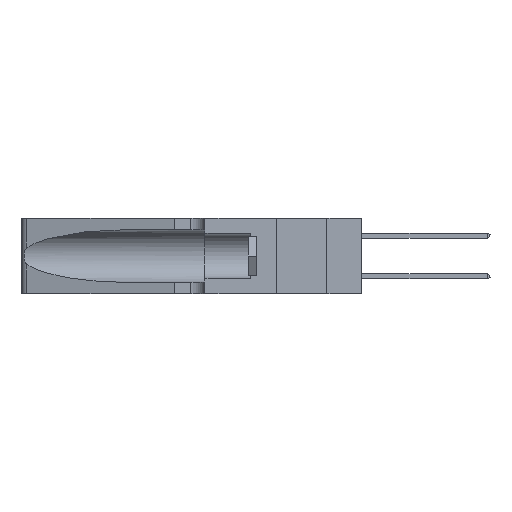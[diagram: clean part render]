
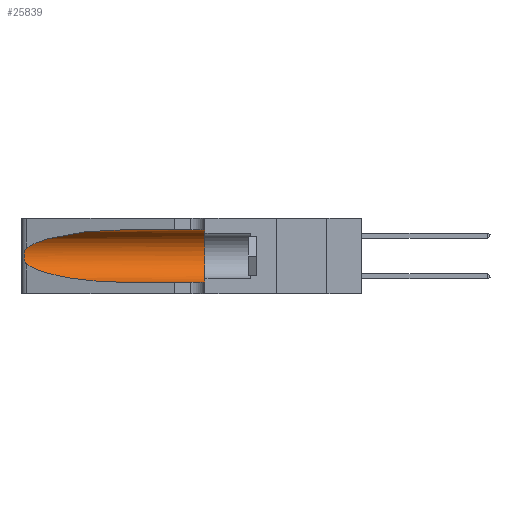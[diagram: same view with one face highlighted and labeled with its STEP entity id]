
A CAD part, left-side view. The second image highlights one B-rep face of the part: STEP entity #25839.
In plain terms, the highlighted cylindrical face has radius 3.308 mm (diameter 6.617 mm), a partial arc.
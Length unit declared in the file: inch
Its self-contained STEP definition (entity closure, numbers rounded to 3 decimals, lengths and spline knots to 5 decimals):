
#1221 = CARTESIAN_POINT ( 'NONE',  ( 0.2373, 1.15595, 0.28018 ) ) ;
#1603 = DIRECTION ( 'NONE',  ( 0., 0., -1. ) ) ;
#2763 = CARTESIAN_POINT ( 'NONE',  ( 0.25854, 1.2359, 0.20912 ) ) ;
#2791 = DIRECTION ( 'NONE',  ( 0., -1., 0. ) ) ;
#3353 = EDGE_LOOP ( 'NONE', ( #34575, #12741, #36280, #5280, #34317, #18163 ) ) ;
#5280 = ORIENTED_EDGE ( 'NONE', *, *, #8085, .T. ) ;
#5352 = VECTOR ( 'NONE', #2791, 39.37008 ) ;
#5541 = VERTEX_POINT ( 'NONE', #17304 ) ;
#5722 = CARTESIAN_POINT ( 'NONE',  ( 0.26075, 1.23896, 0.19203 ) ) ;
#5919 = VERTEX_POINT ( 'NONE', #10292 ) ;
#7194 = FACE_OUTER_BOUND ( 'NONE', #3353, .T. ) ;
#7233 = CARTESIAN_POINT ( 'NONE',  ( 0.1305, 0.35, 0.185 ) ) ;
#7387 = CARTESIAN_POINT ( 'NONE',  ( 0.1305, 1.61858, 0.185 ) ) ;
#7437 = CARTESIAN_POINT ( 'NONE',  ( 0.2373, 1.15595, 0.08982 ) ) ;
#8085 = EDGE_CURVE ( 'NONE', #14605, #11757, #35796, .T. ) ;
#8631 = CARTESIAN_POINT ( 'NONE',  ( 0.26017, 1.23833, 0.17102 ) ) ;
#9462 = VERTEX_POINT ( 'NONE', #19540 ) ;
#10022 = AXIS2_PLACEMENT_3D ( 'NONE', #7233, #27275, #10128 ) ;
#10128 = DIRECTION ( 'NONE',  ( 0., 0., 1. ) ) ;
#10292 = CARTESIAN_POINT ( 'NONE',  ( 0.1305, 0.72297, 0.31525 ) ) ;
#11532 = CARTESIAN_POINT ( 'NONE',  ( 0.25789, 1.23486, 0.15765 ) ) ;
#11757 = VERTEX_POINT ( 'NONE', #12048 ) ;
#12048 = CARTESIAN_POINT ( 'NONE',  ( 0.1305, 0.35, 0.05475 ) ) ;
#12410 =( BOUNDED_CURVE ( )  B_SPLINE_CURVE ( 3, ( #18525, #18650, #1221, #21511 ),
 .UNSPECIFIED., .F., .F. ) 
 B_SPLINE_CURVE_WITH_KNOTS ( ( 4, 4 ),
 ( 1.5708, 2.84003 ),
 .UNSPECIFIED. ) 
 CURVE ( )  GEOMETRIC_REPRESENTATION_ITEM ( )  RATIONAL_B_SPLINE_CURVE ( ( 1., 0.87, 0.87, 1. ) ) 
 REPRESENTATION_ITEM ( '' )  );
#12741 = ORIENTED_EDGE ( 'NONE', *, *, #26076, .T. ) ;
#13222 = CARTESIAN_POINT ( 'NONE',  ( 0.18966, 0.96281, 0.05475 ) ) ;
#13614 = VECTOR ( 'NONE', #18377, 39.37008 ) ;
#14466 = CARTESIAN_POINT ( 'NONE',  ( 0.25555, 1.22993, 0.14849 ) ) ;
#14517 = CARTESIAN_POINT ( 'NONE',  ( 0.1305, 0.72297, 0.05475 ) ) ;
#14605 = VERTEX_POINT ( 'NONE', #14517 ) ;
#17304 = CARTESIAN_POINT ( 'NONE',  ( 0.25487, 1.22718, 0.22369 ) ) ;
#18020 =( BOUNDED_CURVE ( )  B_SPLINE_CURVE ( 3, ( #27490, #7437, #13222, #33171 ),
 .UNSPECIFIED., .F., .F. ) 
 B_SPLINE_CURVE_WITH_KNOTS ( ( 4, 4 ),
 ( 3.44316, 4.71239 ),
 .UNSPECIFIED. ) 
 CURVE ( )  GEOMETRIC_REPRESENTATION_ITEM ( )  RATIONAL_B_SPLINE_CURVE ( ( 1., 0.87, 0.87, 1. ) ) 
 REPRESENTATION_ITEM ( '' )  );
#18163 = ORIENTED_EDGE ( 'NONE', *, *, #24277, .F. ) ;
#18377 = DIRECTION ( 'NONE',  ( 0., -1., 0. ) ) ;
#18525 = CARTESIAN_POINT ( 'NONE',  ( 0.1305, 0.72297, 0.31525 ) ) ;
#18650 = CARTESIAN_POINT ( 'NONE',  ( 0.18966, 0.96281, 0.31525 ) ) ;
#19540 = CARTESIAN_POINT ( 'NONE',  ( 0.1305, 0.35, 0.31525 ) ) ;
#20109 = CARTESIAN_POINT ( 'NONE',  ( 0.25787, 1.23484, 0.2124 ) ) ;
#21511 = CARTESIAN_POINT ( 'NONE',  ( 0.25487, 1.22718, 0.22369 ) ) ;
#21526 = CARTESIAN_POINT ( 'NONE',  ( 0.25487, 1.22718, 0.14631 ) ) ;
#21610 = CYLINDRICAL_SURFACE ( 'NONE', #28870, 0.13025 ) ;
#22972 = CARTESIAN_POINT ( 'NONE',  ( 0.26018, 1.23835, 0.19895 ) ) ;
#23154 = EDGE_CURVE ( 'NONE', #23663, #14605, #18020, .T. ) ;
#23663 = VERTEX_POINT ( 'NONE', #21526 ) ;
#24277 = EDGE_CURVE ( 'NONE', #5919, #9462, #35481, .T. ) ;
#25813 = CARTESIAN_POINT ( 'NONE',  ( 0.26075, 1.23896, 0.178 ) ) ;
#25839 = ADVANCED_FACE ( 'NONE', ( #7194 ), #21610, .F. ) ;
#26076 = EDGE_CURVE ( 'NONE', #5541, #23663, #35783, .T. ) ;
#27275 = DIRECTION ( 'NONE',  ( 0., 1., 0. ) ) ;
#27490 = CARTESIAN_POINT ( 'NONE',  ( 0.25487, 1.22718, 0.14631 ) ) ;
#28556 = CARTESIAN_POINT ( 'NONE',  ( 0.25555, 1.22994, 0.2215 ) ) ;
#28689 = CARTESIAN_POINT ( 'NONE',  ( 0.25856, 1.23593, 0.16098 ) ) ;
#28870 = AXIS2_PLACEMENT_3D ( 'NONE', #7387, #33123, #1603 ) ;
#28955 = EDGE_CURVE ( 'NONE', #5919, #5541, #12410, .T. ) ;
#30147 = CIRCLE ( 'NONE', #10022, 0.13025 ) ;
#31515 = CARTESIAN_POINT ( 'NONE',  ( 0.25639, 1.23186, 0.15144 ) ) ;
#32514 = CARTESIAN_POINT ( 'NONE',  ( 0.1305, 1.61858, 0.31525 ) ) ;
#33123 = DIRECTION ( 'NONE',  ( 0., -1., 0. ) ) ;
#33171 = CARTESIAN_POINT ( 'NONE',  ( 0.1305, 0.72297, 0.05475 ) ) ;
#34137 = CARTESIAN_POINT ( 'NONE',  ( 0.25487, 1.22718, 0.22369 ) ) ;
#34288 = CARTESIAN_POINT ( 'NONE',  ( 0.1305, 1.61858, 0.05475 ) ) ;
#34317 = ORIENTED_EDGE ( 'NONE', *, *, #35138, .F. ) ;
#34380 = CARTESIAN_POINT ( 'NONE',  ( 0.25487, 1.22718, 0.14631 ) ) ;
#34575 = ORIENTED_EDGE ( 'NONE', *, *, #28955, .T. ) ;
#35138 = EDGE_CURVE ( 'NONE', #9462, #11757, #30147, .T. ) ;
#35481 = LINE ( 'NONE', #32514, #13614 ) ;
#35783 = B_SPLINE_CURVE_WITH_KNOTS ( 'NONE', 3,
 ( #34137, #28556, #37089, #20109, #2763, #22972, #5722, #25813, #8631, #28689, #11532, #31515, #14466, #34380 ),
 .UNSPECIFIED., .F., .F.,
 ( 4, 2, 2, 2, 2, 2, 4 ),
 ( 0., 0.00027, 0.00053, 0.00107, 0.0016, 0.00187, 0.00214 ),
 .UNSPECIFIED. ) ;
#35796 = LINE ( 'NONE', #34288, #5352 ) ;
#36280 = ORIENTED_EDGE ( 'NONE', *, *, #23154, .T. ) ;
#37089 = CARTESIAN_POINT ( 'NONE',  ( 0.25639, 1.23184, 0.21858 ) ) ;
